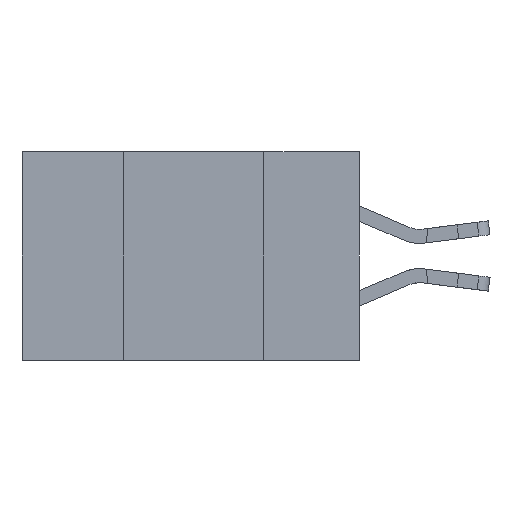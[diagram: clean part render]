
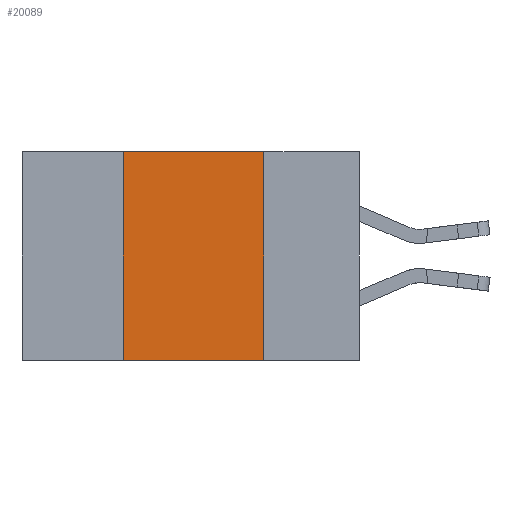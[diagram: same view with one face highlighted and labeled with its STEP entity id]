
A CAD part, left-side view. The second image highlights one B-rep face of the part: STEP entity #20089.
In plain terms, the highlighted planar face has unit normal (-1, 0, 0).
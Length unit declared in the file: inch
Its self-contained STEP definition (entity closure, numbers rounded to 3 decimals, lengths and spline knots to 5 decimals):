
#543 = CARTESIAN_POINT ( 'NONE',  ( 0., 0.17, -0.37 ) ) ;
#753 = LINE ( 'NONE', #3500, #4993 ) ;
#1600 = EDGE_CURVE ( 'NONE', #18872, #16722, #14426, .T. ) ;
#1687 = AXIS2_PLACEMENT_3D ( 'NONE', #2987, #15725, #4855 ) ;
#2987 = CARTESIAN_POINT ( 'NONE',  ( 0., 0.6, 0. ) ) ;
#3500 = CARTESIAN_POINT ( 'NONE',  ( 0., 0.6, 0. ) ) ;
#4173 = DIRECTION ( 'NONE',  ( 0., 0., -1. ) ) ;
#4354 = LINE ( 'NONE', #20309, #13472 ) ;
#4433 = DIRECTION ( 'NONE',  ( 0., -1., 0. ) ) ;
#4607 = ORIENTED_EDGE ( 'NONE', *, *, #10690, .F. ) ;
#4855 = DIRECTION ( 'NONE',  ( 0., 0., -1. ) ) ;
#4993 = VECTOR ( 'NONE', #14427, 39.37008 ) ;
#5044 = VECTOR ( 'NONE', #4173, 39.37008 ) ;
#5065 = CARTESIAN_POINT ( 'NONE',  ( 0., 0.42, -0.37 ) ) ;
#5426 = EDGE_CURVE ( 'NONE', #15141, #12059, #753, .T. ) ;
#9556 = VECTOR ( 'NONE', #4433, 39.37008 ) ;
#10690 = EDGE_CURVE ( 'NONE', #12059, #16722, #15844, .T. ) ;
#11676 = CARTESIAN_POINT ( 'NONE',  ( 0., 0.6, -0.37 ) ) ;
#12059 = VERTEX_POINT ( 'NONE', #19258 ) ;
#12306 = ORIENTED_EDGE ( 'NONE', *, *, #1600, .T. ) ;
#13242 = CARTESIAN_POINT ( 'NONE',  ( 0., 0.17, 0. ) ) ;
#13472 = VECTOR ( 'NONE', #22103, 39.37008 ) ;
#13933 = PLANE ( 'NONE',  #1687 ) ;
#14020 = EDGE_LOOP ( 'NONE', ( #4607, #19080, #16542, #12306 ) ) ;
#14021 = EDGE_CURVE ( 'NONE', #18872, #15141, #4354, .T. ) ;
#14426 = LINE ( 'NONE', #11676, #9556 ) ;
#14427 = DIRECTION ( 'NONE',  ( 0., -1., 0. ) ) ;
#14744 = CARTESIAN_POINT ( 'NONE',  ( 0., 0.42, 0. ) ) ;
#15141 = VERTEX_POINT ( 'NONE', #14744 ) ;
#15372 = FACE_OUTER_BOUND ( 'NONE', #14020, .T. ) ;
#15725 = DIRECTION ( 'NONE',  ( 1., 0., 0. ) ) ;
#15844 = LINE ( 'NONE', #13242, #5044 ) ;
#16542 = ORIENTED_EDGE ( 'NONE', *, *, #14021, .F. ) ;
#16722 = VERTEX_POINT ( 'NONE', #543 ) ;
#18872 = VERTEX_POINT ( 'NONE', #5065 ) ;
#19080 = ORIENTED_EDGE ( 'NONE', *, *, #5426, .F. ) ;
#19258 = CARTESIAN_POINT ( 'NONE',  ( 0., 0.17, 0. ) ) ;
#20089 = ADVANCED_FACE ( 'NONE', ( #15372 ), #13933, .F. ) ;
#20309 = CARTESIAN_POINT ( 'NONE',  ( 0., 0.42, 0. ) ) ;
#22103 = DIRECTION ( 'NONE',  ( 0., 0., 1. ) ) ;
